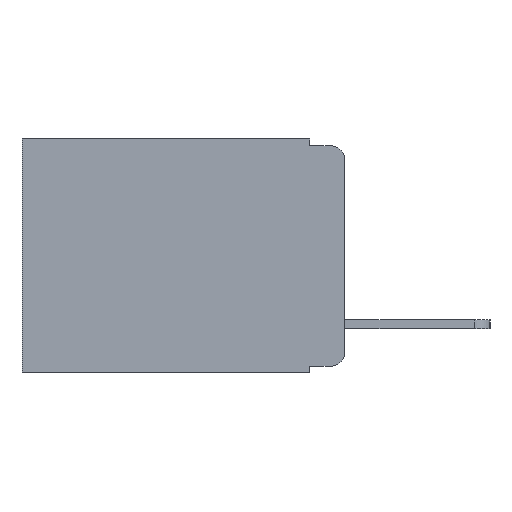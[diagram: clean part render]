
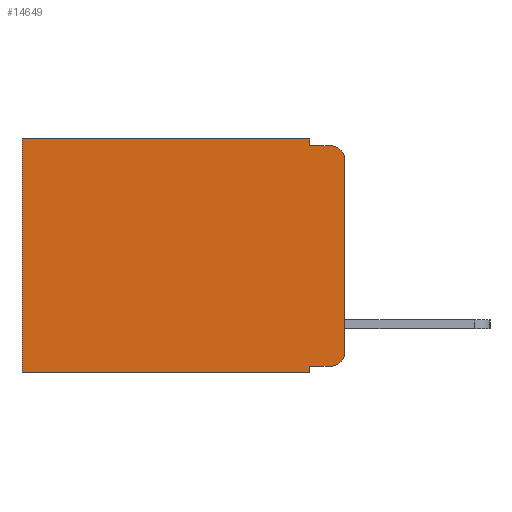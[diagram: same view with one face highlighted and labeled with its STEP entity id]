
A CAD part, left-side view. The second image highlights one B-rep face of the part: STEP entity #14649.
In plain terms, the highlighted planar face has unit normal (-1, 0, 0).
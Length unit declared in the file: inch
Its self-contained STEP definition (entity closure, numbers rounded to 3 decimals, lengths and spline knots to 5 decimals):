
#12 = EDGE_CURVE ( 'NONE', #20179, #20722, #3736, .T. ) ;
#99 = EDGE_CURVE ( 'NONE', #20179, #10455, #10833, .T. ) ;
#127 = EDGE_CURVE ( 'NONE', #6916, #10455, #18791, .T. ) ;
#237 = EDGE_CURVE ( 'NONE', #775, #6916, #2926, .T. ) ;
#293 = EDGE_CURVE ( 'NONE', #775, #21763, #15117, .T. ) ;
#313 = EDGE_CURVE ( 'NONE', #21763, #9663, #5372, .T. ) ;
#354 = EDGE_CURVE ( 'NONE', #10963, #8405, #13498, .T. ) ;
#381 = EDGE_CURVE ( 'NONE', #10963, #13606, #16974, .T. ) ;
#451 = EDGE_CURVE ( 'NONE', #13606, #20722, #11365, .T. ) ;
#775 = VERTEX_POINT ( 'NONE', #14094 ) ;
#1170 = DIRECTION ( 'NONE',  ( 0., 0., -1. ) ) ;
#1184 = VECTOR ( 'NONE', #18287, 39.37008 ) ;
#1745 = PLANE ( 'NONE',  #13029 ) ;
#2343 = DIRECTION ( 'NONE',  ( 0., 0., -1. ) ) ;
#2351 = VECTOR ( 'NONE', #10368, 39.37008 ) ;
#2926 = LINE ( 'NONE', #8330, #2351 ) ;
#3383 = ORIENTED_EDGE ( 'NONE', *, *, #237, .F. ) ;
#3521 = DIRECTION ( 'NONE',  ( 1., 0., 0. ) ) ;
#3715 = VECTOR ( 'NONE', #19076, 39.37008 ) ;
#3736 = LINE ( 'NONE', #7297, #16485 ) ;
#4618 = CARTESIAN_POINT ( 'NONE',  ( 0.298, 0., 0. ) ) ;
#5372 = LINE ( 'NONE', #11948, #14009 ) ;
#6203 = CARTESIAN_POINT ( 'NONE',  ( 0.298, 0.02, -0.313 ) ) ;
#6916 = VERTEX_POINT ( 'NONE', #17821 ) ;
#6989 = ORIENTED_EDGE ( 'NONE', *, *, #12, .F. ) ;
#7015 = CARTESIAN_POINT ( 'NONE',  ( 0.298, 0.02, -0.333 ) ) ;
#7297 = CARTESIAN_POINT ( 'NONE',  ( 0.298, 0., 0. ) ) ;
#8084 = ORIENTED_EDGE ( 'NONE', *, *, #293, .T. ) ;
#8116 = CARTESIAN_POINT ( 'NONE',  ( 0.298, 0.02, -0.01 ) ) ;
#8330 = CARTESIAN_POINT ( 'NONE',  ( 0.298, 0.051, 0. ) ) ;
#8405 = VERTEX_POINT ( 'NONE', #18147 ) ;
#8536 = CARTESIAN_POINT ( 'NONE',  ( 0.298, 0.473, -0.343 ) ) ;
#8759 = CARTESIAN_POINT ( 'NONE',  ( 0.298, 0.051, -0.01 ) ) ;
#9237 = EDGE_CURVE ( 'NONE', #8405, #9663, #15281, .T. ) ;
#9663 = VERTEX_POINT ( 'NONE', #8536 ) ;
#9889 = CARTESIAN_POINT ( 'NONE',  ( 0.298, 0.051, -0.333 ) ) ;
#10368 = DIRECTION ( 'NONE',  ( 0., 0., -1. ) ) ;
#10455 = VERTEX_POINT ( 'NONE', #8116 ) ;
#10770 = EDGE_LOOP ( 'NONE', ( #6989, #16133, #21050, #3383, #8084, #13167, #19222, #19748, #16425, #20801 ) ) ;
#10833 = CIRCLE ( 'NONE', #16049, 0.02 ) ;
#10963 = VERTEX_POINT ( 'NONE', #9889 ) ;
#11032 = AXIS2_PLACEMENT_3D ( 'NONE', #6203, #17117, #13426 ) ;
#11365 = CIRCLE ( 'NONE', #11032, 0.02 ) ;
#11948 = CARTESIAN_POINT ( 'NONE',  ( 0.298, 0.473, 0. ) ) ;
#12591 = CARTESIAN_POINT ( 'NONE',  ( 0.298, 0.473, 0. ) ) ;
#13029 = AXIS2_PLACEMENT_3D ( 'NONE', #13898, #3521, #15656 ) ;
#13167 = ORIENTED_EDGE ( 'NONE', *, *, #313, .T. ) ;
#13420 = FACE_OUTER_BOUND ( 'NONE', #10770, .T. ) ;
#13426 = DIRECTION ( 'NONE',  ( 0., 0., -1. ) ) ;
#13498 = LINE ( 'NONE', #19114, #3715 ) ;
#13606 = VERTEX_POINT ( 'NONE', #7015 ) ;
#13891 = DIRECTION ( 'NONE',  ( -1., 0., 0. ) ) ;
#13898 = CARTESIAN_POINT ( 'NONE',  ( 0.298, 0., 0. ) ) ;
#14009 = VECTOR ( 'NONE', #2343, 39.37008 ) ;
#14094 = CARTESIAN_POINT ( 'NONE',  ( 0.298, 0.051, 0. ) ) ;
#14215 = CARTESIAN_POINT ( 'NONE',  ( 0.298, 0.02, -0.03 ) ) ;
#14649 = ADVANCED_FACE ( 'NONE', ( #13420 ), #1745, .F. ) ;
#15117 = LINE ( 'NONE', #4618, #1184 ) ;
#15281 = LINE ( 'NONE', #17839, #19183 ) ;
#15446 = CARTESIAN_POINT ( 'NONE',  ( 0.298, 0.051, -0.333 ) ) ;
#15656 = DIRECTION ( 'NONE',  ( 0., 0., -1. ) ) ;
#15952 = DIRECTION ( 'NONE',  ( 0., -1., 0. ) ) ;
#16049 = AXIS2_PLACEMENT_3D ( 'NONE', #14215, #13891, #16773 ) ;
#16133 = ORIENTED_EDGE ( 'NONE', *, *, #99, .T. ) ;
#16170 = DIRECTION ( 'NONE',  ( 0., 1., 0. ) ) ;
#16425 = ORIENTED_EDGE ( 'NONE', *, *, #381, .T. ) ;
#16485 = VECTOR ( 'NONE', #1170, 39.37008 ) ;
#16773 = DIRECTION ( 'NONE',  ( 0., 0., -1. ) ) ;
#16974 = LINE ( 'NONE', #15446, #17485 ) ;
#17117 = DIRECTION ( 'NONE',  ( -1., 0., 0. ) ) ;
#17417 = DIRECTION ( 'NONE',  ( 0., -1., 0. ) ) ;
#17485 = VECTOR ( 'NONE', #17417, 39.37008 ) ;
#17821 = CARTESIAN_POINT ( 'NONE',  ( 0.298, 0.051, -0.01 ) ) ;
#17839 = CARTESIAN_POINT ( 'NONE',  ( 0.298, 0., -0.343 ) ) ;
#17851 = CARTESIAN_POINT ( 'NONE',  ( 0.298, 0., -0.03 ) ) ;
#18147 = CARTESIAN_POINT ( 'NONE',  ( 0.298, 0.051, -0.343 ) ) ;
#18287 = DIRECTION ( 'NONE',  ( 0., 1., 0. ) ) ;
#18289 = VECTOR ( 'NONE', #15952, 39.37008 ) ;
#18791 = LINE ( 'NONE', #8759, #18289 ) ;
#18940 = CARTESIAN_POINT ( 'NONE',  ( 0.298, 0., -0.313 ) ) ;
#19076 = DIRECTION ( 'NONE',  ( 0., 0., -1. ) ) ;
#19114 = CARTESIAN_POINT ( 'NONE',  ( 0.298, 0.051, 0. ) ) ;
#19183 = VECTOR ( 'NONE', #16170, 39.37008 ) ;
#19222 = ORIENTED_EDGE ( 'NONE', *, *, #9237, .F. ) ;
#19748 = ORIENTED_EDGE ( 'NONE', *, *, #354, .F. ) ;
#20179 = VERTEX_POINT ( 'NONE', #17851 ) ;
#20722 = VERTEX_POINT ( 'NONE', #18940 ) ;
#20801 = ORIENTED_EDGE ( 'NONE', *, *, #451, .T. ) ;
#21050 = ORIENTED_EDGE ( 'NONE', *, *, #127, .F. ) ;
#21763 = VERTEX_POINT ( 'NONE', #12591 ) ;
